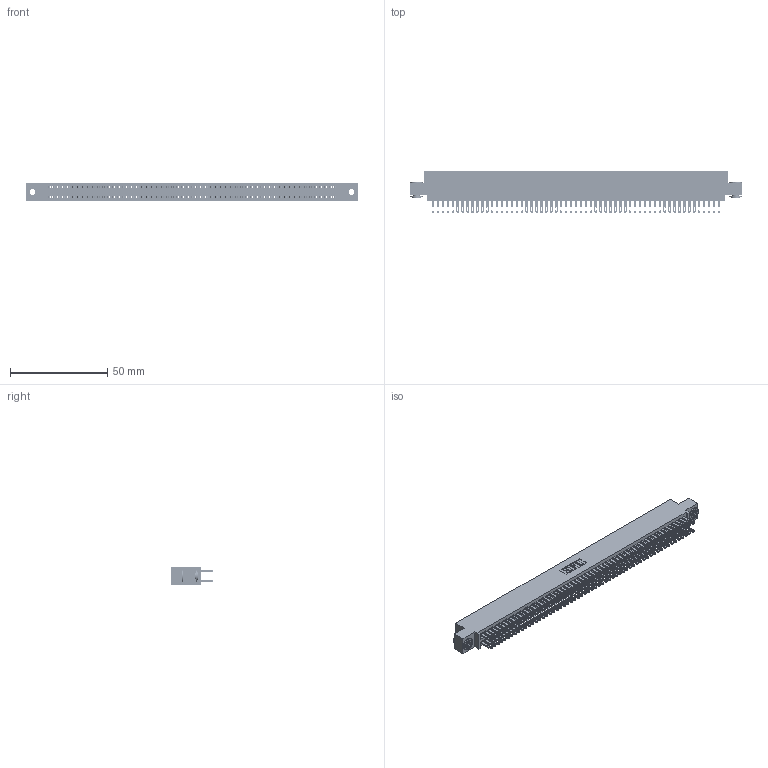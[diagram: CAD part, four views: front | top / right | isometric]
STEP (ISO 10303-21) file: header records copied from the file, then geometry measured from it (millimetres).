
FILE_DESCRIPTION (( 'STEP AP203' ), '1' );
FILE_NAME ('895-118-500-503.STEP', '2020-10-13T14:37:37', ( '' ), ( '' ), 'SwSTEP 2.0', 'SolidWorks 2020', '' );
FILE_SCHEMA (( 'CONFIG_CONTROL_DESIGN' ));
Length unit declared in the file: inch
Products named in the file (4): 845 Part_0.110 Offset - 0.156 Dia-TH; 345-250-002_345-250-002-102; 345-292-001_345-293-100; 895-118-500-503
Assembly tree (121 placements, depth 2):
  895-118-500-503
    845 Part_0.110 Offset - 0.156 Dia-TH
    345-292-001_345-293-100  x118
    345-250-002_345-250-002-102  x2
Bounding box: 171.07 x 21.51 x 9.4 mm (x, y, z)
Volume: 17082.2 mm3; surface area: 27080.9 mm2
Topology: 121 solids, 121 shells, 5596 faces, 17067 edges, 11374 vertices
Faces by surface type: plane 3280, cylinder 2308, cone 8
Entity records: 44716 total; most frequent: CARTESIAN_POINT 7455, ORIENTED_EDGE 7382, DIRECTION 6585, EDGE_CURVE 3691, VECTOR 3295, LINE 3295, VERTEX_POINT 2458, AXIS2_PLACEMENT_3D 1645
